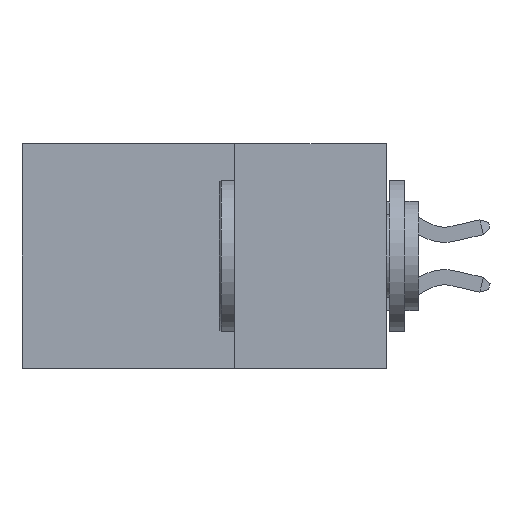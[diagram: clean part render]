
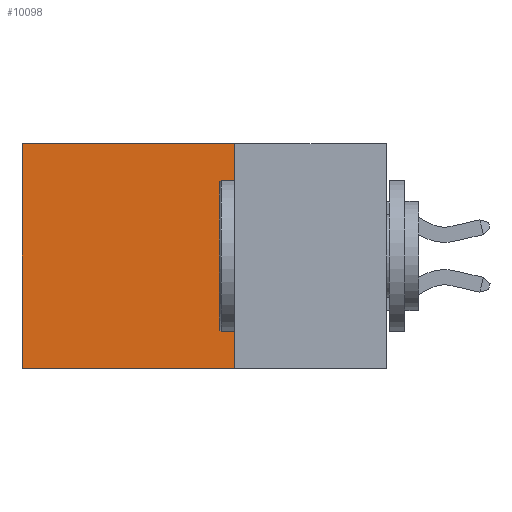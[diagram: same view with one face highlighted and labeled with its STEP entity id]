
A CAD part, left-side view. The second image highlights one B-rep face of the part: STEP entity #10098.
In plain terms, the highlighted planar face has unit normal (-1, 0, 0).
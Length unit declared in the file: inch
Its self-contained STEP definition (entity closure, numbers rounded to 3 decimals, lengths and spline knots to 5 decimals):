
#360 = LINE ( 'NONE', #1814, #4146 ) ;
#1132 = PLANE ( 'NONE',  #22001 ) ;
#1164 = EDGE_LOOP ( 'NONE', ( #3664, #19394, #1395, #21358 ) ) ;
#1286 = VERTEX_POINT ( 'NONE', #16902 ) ;
#1395 = ORIENTED_EDGE ( 'NONE', *, *, #20730, .F. ) ;
#1512 = LINE ( 'NONE', #11689, #18587 ) ;
#1814 = CARTESIAN_POINT ( 'NONE',  ( 0.298, 0.25, -0.37 ) ) ;
#2251 = VERTEX_POINT ( 'NONE', #13433 ) ;
#3229 = DIRECTION ( 'NONE',  ( 0., 0., -1. ) ) ;
#3664 = ORIENTED_EDGE ( 'NONE', *, *, #25964, .T. ) ;
#4146 = VECTOR ( 'NONE', #10444, 39.37008 ) ;
#5063 = CARTESIAN_POINT ( 'NONE',  ( 0.298, 0.25, -0.37 ) ) ;
#5095 = DIRECTION ( 'NONE',  ( 0., 0., -1. ) ) ;
#5249 = CARTESIAN_POINT ( 'NONE',  ( 0.298, 0.25, 0. ) ) ;
#6491 = EDGE_CURVE ( 'NONE', #25462, #1286, #360, .T. ) ;
#10098 = ADVANCED_FACE ( 'NONE', ( #21638 ), #1132, .F. ) ;
#10444 = DIRECTION ( 'NONE',  ( 0., 1., 0. ) ) ;
#10960 = VECTOR ( 'NONE', #22099, 39.37008 ) ;
#11689 = CARTESIAN_POINT ( 'NONE',  ( 0.298, 0.6, 0. ) ) ;
#13433 = CARTESIAN_POINT ( 'NONE',  ( 0.298, 0.25, 0. ) ) ;
#14167 = EDGE_CURVE ( 'NONE', #2251, #27772, #19161, .T. ) ;
#15156 = LINE ( 'NONE', #18153, #18228 ) ;
#15319 = CARTESIAN_POINT ( 'NONE',  ( 0.298, 0.6, 0. ) ) ;
#16300 = DIRECTION ( 'NONE',  ( 1., 0., 0. ) ) ;
#16902 = CARTESIAN_POINT ( 'NONE',  ( 0.298, 0.6, -0.37 ) ) ;
#18153 = CARTESIAN_POINT ( 'NONE',  ( 0.298, 0.25, 0. ) ) ;
#18228 = VECTOR ( 'NONE', #5095, 39.37008 ) ;
#18587 = VECTOR ( 'NONE', #26973, 39.37008 ) ;
#19161 = LINE ( 'NONE', #26806, #10960 ) ;
#19394 = ORIENTED_EDGE ( 'NONE', *, *, #6491, .F. ) ;
#20730 = EDGE_CURVE ( 'NONE', #2251, #25462, #15156, .T. ) ;
#21358 = ORIENTED_EDGE ( 'NONE', *, *, #14167, .T. ) ;
#21638 = FACE_OUTER_BOUND ( 'NONE', #1164, .T. ) ;
#22001 = AXIS2_PLACEMENT_3D ( 'NONE', #5249, #16300, #3229 ) ;
#22099 = DIRECTION ( 'NONE',  ( 0., 1., 0. ) ) ;
#25462 = VERTEX_POINT ( 'NONE', #5063 ) ;
#25964 = EDGE_CURVE ( 'NONE', #27772, #1286, #1512, .T. ) ;
#26806 = CARTESIAN_POINT ( 'NONE',  ( 0.298, 0.25, 0. ) ) ;
#26973 = DIRECTION ( 'NONE',  ( 0., 0., -1. ) ) ;
#27772 = VERTEX_POINT ( 'NONE', #15319 ) ;
